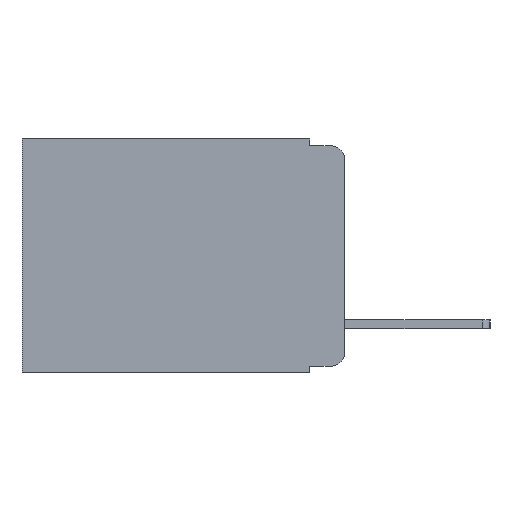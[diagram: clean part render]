
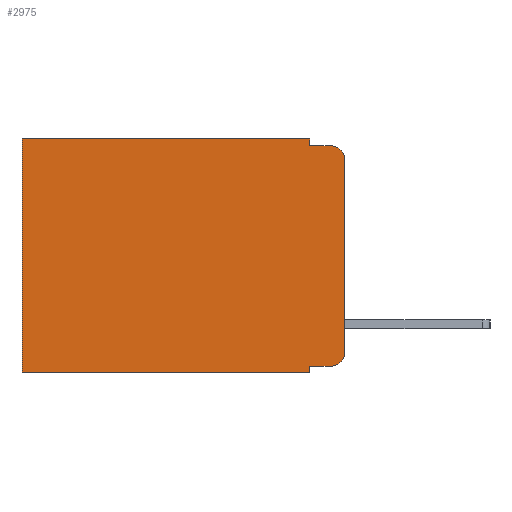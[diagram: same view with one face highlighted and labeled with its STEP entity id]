
A CAD part, left-side view. The second image highlights one B-rep face of the part: STEP entity #2975.
In plain terms, the highlighted planar face has unit normal (-1, 0, 0).
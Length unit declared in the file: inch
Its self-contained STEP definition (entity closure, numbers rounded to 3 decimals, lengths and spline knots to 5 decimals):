
#14 = DIRECTION ( 'NONE',  ( -1., 0., 0. ) ) ;
#110 = DIRECTION ( 'NONE',  ( 0., 0., -1. ) ) ;
#698 = DIRECTION ( 'NONE',  ( 0., 0., -1. ) ) ;
#756 = VECTOR ( 'NONE', #817, 39.37008 ) ;
#784 = CARTESIAN_POINT ( 'NONE',  ( 0.298, 0.02, -0.03 ) ) ;
#789 = CARTESIAN_POINT ( 'NONE',  ( 0.298, 0.473, 0. ) ) ;
#817 = DIRECTION ( 'NONE',  ( 0., 0., -1. ) ) ;
#911 = EDGE_CURVE ( 'NONE', #6491, #2515, #3143, .T. ) ;
#1418 = EDGE_CURVE ( 'NONE', #8445, #20837, #14206, .T. ) ;
#1549 = ORIENTED_EDGE ( 'NONE', *, *, #1963, .F. ) ;
#1887 = EDGE_CURVE ( 'NONE', #20911, #5939, #14962, .T. ) ;
#1897 = EDGE_CURVE ( 'NONE', #20911, #3790, #5750, .T. ) ;
#1922 = EDGE_CURVE ( 'NONE', #5072, #3790, #18686, .T. ) ;
#1924 = EDGE_CURVE ( 'NONE', #6491, #5072, #9882, .T. ) ;
#1927 = EDGE_CURVE ( 'NONE', #2515, #20837, #13898, .T. ) ;
#1942 = CARTESIAN_POINT ( 'NONE',  ( 0.298, 0., -0.343 ) ) ;
#1963 = EDGE_CURVE ( 'NONE', #11486, #8445, #7664, .T. ) ;
#1985 = EDGE_CURVE ( 'NONE', #11486, #5871, #19909, .T. ) ;
#1997 = EDGE_CURVE ( 'NONE', #5871, #5939, #15699, .T. ) ;
#2130 = ORIENTED_EDGE ( 'NONE', *, *, #1985, .T. ) ;
#2515 = VERTEX_POINT ( 'NONE', #15818 ) ;
#2803 = ORIENTED_EDGE ( 'NONE', *, *, #1887, .F. ) ;
#2975 = ADVANCED_FACE ( 'NONE', ( #8742 ), #18048, .F. ) ;
#3143 = LINE ( 'NONE', #14400, #12547 ) ;
#3250 = CARTESIAN_POINT ( 'NONE',  ( 0.298, 0.02, -0.333 ) ) ;
#3790 = VERTEX_POINT ( 'NONE', #5098 ) ;
#3817 = ORIENTED_EDGE ( 'NONE', *, *, #1997, .T. ) ;
#4600 = VECTOR ( 'NONE', #9358, 39.37008 ) ;
#5072 = VERTEX_POINT ( 'NONE', #6256 ) ;
#5098 = CARTESIAN_POINT ( 'NONE',  ( 0.298, 0.02, -0.01 ) ) ;
#5184 = VECTOR ( 'NONE', #10040, 39.37008 ) ;
#5396 = CARTESIAN_POINT ( 'NONE',  ( 0.298, 0., 0. ) ) ;
#5750 = CIRCLE ( 'NONE', #6325, 0.02 ) ;
#5871 = VERTEX_POINT ( 'NONE', #3250 ) ;
#5939 = VERTEX_POINT ( 'NONE', #17396 ) ;
#6070 = DIRECTION ( 'NONE',  ( -1., 0., 0. ) ) ;
#6091 = ORIENTED_EDGE ( 'NONE', *, *, #1924, .F. ) ;
#6123 = CARTESIAN_POINT ( 'NONE',  ( 0.298, 0.051, -0.333 ) ) ;
#6174 = ORIENTED_EDGE ( 'NONE', *, *, #911, .T. ) ;
#6256 = CARTESIAN_POINT ( 'NONE',  ( 0.298, 0.051, -0.01 ) ) ;
#6325 = AXIS2_PLACEMENT_3D ( 'NONE', #784, #14, #110 ) ;
#6332 = ORIENTED_EDGE ( 'NONE', *, *, #1418, .F. ) ;
#6491 = VERTEX_POINT ( 'NONE', #7436 ) ;
#6632 = CARTESIAN_POINT ( 'NONE',  ( 0.298, 0.02, -0.313 ) ) ;
#6659 = ORIENTED_EDGE ( 'NONE', *, *, #1927, .T. ) ;
#6685 = DIRECTION ( 'NONE',  ( 0., 0., -1. ) ) ;
#6784 = ORIENTED_EDGE ( 'NONE', *, *, #1922, .F. ) ;
#7342 = ORIENTED_EDGE ( 'NONE', *, *, #1897, .T. ) ;
#7436 = CARTESIAN_POINT ( 'NONE',  ( 0.298, 0.051, 0. ) ) ;
#7576 = CARTESIAN_POINT ( 'NONE',  ( 0.298, 0.473, -0.343 ) ) ;
#7664 = LINE ( 'NONE', #21256, #20391 ) ;
#8445 = VERTEX_POINT ( 'NONE', #20615 ) ;
#8742 = FACE_OUTER_BOUND ( 'NONE', #10719, .T. ) ;
#9240 = AXIS2_PLACEMENT_3D ( 'NONE', #5396, #17009, #16870 ) ;
#9358 = DIRECTION ( 'NONE',  ( 0., 0., -1. ) ) ;
#9882 = LINE ( 'NONE', #18179, #4600 ) ;
#10040 = DIRECTION ( 'NONE',  ( 0., -1., 0. ) ) ;
#10719 = EDGE_LOOP ( 'NONE', ( #2803, #7342, #6784, #6091, #6174, #6659, #6332, #1549, #2130, #3817 ) ) ;
#11486 = VERTEX_POINT ( 'NONE', #12560 ) ;
#12547 = VECTOR ( 'NONE', #16319, 39.37008 ) ;
#12560 = CARTESIAN_POINT ( 'NONE',  ( 0.298, 0.051, -0.333 ) ) ;
#13898 = LINE ( 'NONE', #789, #17709 ) ;
#14206 = LINE ( 'NONE', #1942, #17993 ) ;
#14400 = CARTESIAN_POINT ( 'NONE',  ( 0.298, 0., 0. ) ) ;
#14962 = LINE ( 'NONE', #16930, #756 ) ;
#15699 = CIRCLE ( 'NONE', #17655, 0.02 ) ;
#15818 = CARTESIAN_POINT ( 'NONE',  ( 0.298, 0.473, 0. ) ) ;
#16125 = DIRECTION ( 'NONE',  ( 0., -1., 0. ) ) ;
#16217 = VECTOR ( 'NONE', #16125, 39.37008 ) ;
#16319 = DIRECTION ( 'NONE',  ( 0., 1., 0. ) ) ;
#16870 = DIRECTION ( 'NONE',  ( 0., 0., -1. ) ) ;
#16930 = CARTESIAN_POINT ( 'NONE',  ( 0.298, 0., 0. ) ) ;
#17009 = DIRECTION ( 'NONE',  ( 1., 0., 0. ) ) ;
#17396 = CARTESIAN_POINT ( 'NONE',  ( 0.298, 0., -0.313 ) ) ;
#17655 = AXIS2_PLACEMENT_3D ( 'NONE', #6632, #6070, #6685 ) ;
#17709 = VECTOR ( 'NONE', #698, 39.37008 ) ;
#17837 = CARTESIAN_POINT ( 'NONE',  ( 0.298, 0., -0.03 ) ) ;
#17993 = VECTOR ( 'NONE', #21371, 39.37008 ) ;
#18048 = PLANE ( 'NONE',  #9240 ) ;
#18179 = CARTESIAN_POINT ( 'NONE',  ( 0.298, 0.051, 0. ) ) ;
#18402 = CARTESIAN_POINT ( 'NONE',  ( 0.298, 0.051, -0.01 ) ) ;
#18686 = LINE ( 'NONE', #18402, #5184 ) ;
#19909 = LINE ( 'NONE', #6123, #16217 ) ;
#20391 = VECTOR ( 'NONE', #21206, 39.37008 ) ;
#20615 = CARTESIAN_POINT ( 'NONE',  ( 0.298, 0.051, -0.343 ) ) ;
#20837 = VERTEX_POINT ( 'NONE', #7576 ) ;
#20911 = VERTEX_POINT ( 'NONE', #17837 ) ;
#21206 = DIRECTION ( 'NONE',  ( 0., 0., -1. ) ) ;
#21256 = CARTESIAN_POINT ( 'NONE',  ( 0.298, 0.051, 0. ) ) ;
#21371 = DIRECTION ( 'NONE',  ( 0., 1., 0. ) ) ;
